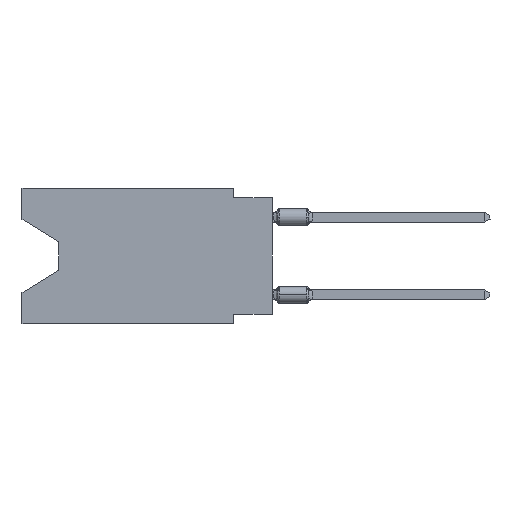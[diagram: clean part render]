
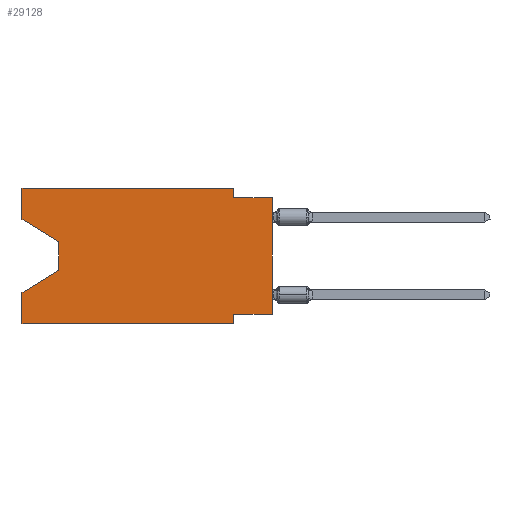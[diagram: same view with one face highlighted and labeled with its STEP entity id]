
A CAD part, left-side view. The second image highlights one B-rep face of the part: STEP entity #29128.
In plain terms, the highlighted planar face has unit normal (-1, 0, 0).
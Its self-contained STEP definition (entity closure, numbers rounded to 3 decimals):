
#544 = CARTESIAN_POINT ( 'NONE',  ( 0., 2.54, -8.89 ) ) ;
#2797 = DIRECTION ( 'NONE',  ( 0., 0., 1. ) ) ;
#3308 = CARTESIAN_POINT ( 'NONE',  ( 0., 0., -0.635 ) ) ;
#3754 = CARTESIAN_POINT ( 'NONE',  ( 0., 2.54, -8.255 ) ) ;
#3986 = CARTESIAN_POINT ( 'NONE',  ( 0., 2.54, -8.89 ) ) ;
#6310 = ORIENTED_EDGE ( 'NONE', *, *, #25514, .T. ) ;
#7129 = ORIENTED_EDGE ( 'NONE', *, *, #29962, .F. ) ;
#7246 = LINE ( 'NONE', #46745, #50646 ) ;
#7918 = VECTOR ( 'NONE', #38647, 1000. ) ;
#8728 = ORIENTED_EDGE ( 'NONE', *, *, #28057, .F. ) ;
#8748 = CARTESIAN_POINT ( 'NONE',  ( 0., 16.383, 0. ) ) ;
#9948 = DIRECTION ( 'NONE',  ( 0., -0.855, -0.519 ) ) ;
#12401 = ORIENTED_EDGE ( 'NONE', *, *, #23514, .T. ) ;
#13628 = CARTESIAN_POINT ( 'NONE',  ( 0., 13.97, -5.385 ) ) ;
#14386 = VECTOR ( 'NONE', #37994, 1000. ) ;
#14815 = VERTEX_POINT ( 'NONE', #20829 ) ;
#14848 = LINE ( 'NONE', #34780, #24782 ) ;
#15289 = EDGE_CURVE ( 'NONE', #25680, #18998, #44597, .T. ) ;
#16782 = VERTEX_POINT ( 'NONE', #3754 ) ;
#17355 = DIRECTION ( 'NONE',  ( 0., 0., 1. ) ) ;
#17491 = CARTESIAN_POINT ( 'NONE',  ( 0., 16.383, -8.89 ) ) ;
#18998 = VERTEX_POINT ( 'NONE', #3308 ) ;
#19132 = ORIENTED_EDGE ( 'NONE', *, *, #34079, .F. ) ;
#19628 = ORIENTED_EDGE ( 'NONE', *, *, #15289, .F. ) ;
#19960 = VECTOR ( 'NONE', #62646, 1000. ) ;
#20457 = DIRECTION ( 'NONE',  ( 0., 0., -1. ) ) ;
#20829 = CARTESIAN_POINT ( 'NONE',  ( 0., 16.383, -8.89 ) ) ;
#22309 = CARTESIAN_POINT ( 'NONE',  ( 0., 0., -8.255 ) ) ;
#22534 = CARTESIAN_POINT ( 'NONE',  ( 0., 0., -8.255 ) ) ;
#23514 = EDGE_CURVE ( 'NONE', #55334, #18998, #26099, .T. ) ;
#24268 = ORIENTED_EDGE ( 'NONE', *, *, #50638, .F. ) ;
#24782 = VECTOR ( 'NONE', #9948, 1000. ) ;
#24988 = CARTESIAN_POINT ( 'NONE',  ( 0., 16.383, -2.038 ) ) ;
#25101 = VECTOR ( 'NONE', #35912, 1000. ) ;
#25110 = LINE ( 'NONE', #17491, #61078 ) ;
#25514 = EDGE_CURVE ( 'NONE', #60971, #62952, #43201, .T. ) ;
#25680 = VERTEX_POINT ( 'NONE', #40229 ) ;
#26099 = LINE ( 'NONE', #62016, #25101 ) ;
#26554 = PLANE ( 'NONE',  #51861 ) ;
#27206 = DIRECTION ( 'NONE',  ( 0., 0., -1. ) ) ;
#27913 = ORIENTED_EDGE ( 'NONE', *, *, #57124, .F. ) ;
#27999 = LINE ( 'NONE', #8748, #52180 ) ;
#28057 = EDGE_CURVE ( 'NONE', #55334, #16782, #47112, .T. ) ;
#29037 = EDGE_CURVE ( 'NONE', #37709, #36708, #14848, .T. ) ;
#29128 = ADVANCED_FACE ( 'NONE', ( #46813 ), #26554, .F. ) ;
#29423 = CARTESIAN_POINT ( 'NONE',  ( 0., 16.383, 0. ) ) ;
#29962 = EDGE_CURVE ( 'NONE', #37709, #45222, #46222, .T. ) ;
#30205 = DIRECTION ( 'NONE',  ( 0., -1., 0. ) ) ;
#31523 = CARTESIAN_POINT ( 'NONE',  ( 0., 16.383, 0. ) ) ;
#32145 = EDGE_CURVE ( 'NONE', #45222, #53547, #27999, .T. ) ;
#32771 = CARTESIAN_POINT ( 'NONE',  ( 0., 16.383, -6.852 ) ) ;
#33240 = DIRECTION ( 'NONE',  ( 0., -1., 0. ) ) ;
#34079 = EDGE_CURVE ( 'NONE', #53547, #25680, #47617, .T. ) ;
#34780 = CARTESIAN_POINT ( 'NONE',  ( 0., 16.383, -2.038 ) ) ;
#35038 = VECTOR ( 'NONE', #17355, 1000. ) ;
#35664 = ORIENTED_EDGE ( 'NONE', *, *, #50561, .T. ) ;
#35912 = DIRECTION ( 'NONE',  ( 0., 0., 1. ) ) ;
#35940 = VECTOR ( 'NONE', #20457, 1000. ) ;
#36708 = VERTEX_POINT ( 'NONE', #44752 ) ;
#37709 = VERTEX_POINT ( 'NONE', #24988 ) ;
#37935 = LINE ( 'NONE', #52620, #35038 ) ;
#37994 = DIRECTION ( 'NONE',  ( 0., 1., 0. ) ) ;
#38647 = DIRECTION ( 'NONE',  ( 0., 0.855, -0.519 ) ) ;
#39609 = VERTEX_POINT ( 'NONE', #3986 ) ;
#40229 = CARTESIAN_POINT ( 'NONE',  ( 0., 2.54, -0.635 ) ) ;
#41081 = DIRECTION ( 'NONE',  ( 0., -1., 0. ) ) ;
#41629 = ORIENTED_EDGE ( 'NONE', *, *, #47003, .T. ) ;
#43131 = VECTOR ( 'NONE', #30205, 1000. ) ;
#43201 = LINE ( 'NONE', #63467, #7918 ) ;
#44597 = LINE ( 'NONE', #45230, #43131 ) ;
#44752 = CARTESIAN_POINT ( 'NONE',  ( 0., 13.97, -3.505 ) ) ;
#45222 = VERTEX_POINT ( 'NONE', #29423 ) ;
#45230 = CARTESIAN_POINT ( 'NONE',  ( 0., 0., -0.635 ) ) ;
#46222 = LINE ( 'NONE', #31523, #50927 ) ;
#46481 = CARTESIAN_POINT ( 'NONE',  ( 0., 16.383, 0. ) ) ;
#46745 = CARTESIAN_POINT ( 'NONE',  ( 0., 13.97, -3.505 ) ) ;
#46813 = FACE_OUTER_BOUND ( 'NONE', #56754, .T. ) ;
#47003 = EDGE_CURVE ( 'NONE', #14815, #39609, #25110, .T. ) ;
#47112 = LINE ( 'NONE', #22309, #14386 ) ;
#47382 = DIRECTION ( 'NONE',  ( 0., 0., -1. ) ) ;
#47617 = LINE ( 'NONE', #53834, #19960 ) ;
#50561 = EDGE_CURVE ( 'NONE', #36708, #60971, #7246, .T. ) ;
#50638 = EDGE_CURVE ( 'NONE', #14815, #62952, #37935, .T. ) ;
#50646 = VECTOR ( 'NONE', #47382, 1000. ) ;
#50927 = VECTOR ( 'NONE', #2797, 1000. ) ;
#51058 = ORIENTED_EDGE ( 'NONE', *, *, #32145, .F. ) ;
#51717 = DIRECTION ( 'NONE',  ( 1., 0., 0. ) ) ;
#51861 = AXIS2_PLACEMENT_3D ( 'NONE', #46481, #51717, #27206 ) ;
#52180 = VECTOR ( 'NONE', #33240, 1000. ) ;
#52620 = CARTESIAN_POINT ( 'NONE',  ( 0., 16.383, 0. ) ) ;
#53547 = VERTEX_POINT ( 'NONE', #59257 ) ;
#53834 = CARTESIAN_POINT ( 'NONE',  ( 0., 2.54, 0. ) ) ;
#54748 = LINE ( 'NONE', #544, #35940 ) ;
#55334 = VERTEX_POINT ( 'NONE', #22534 ) ;
#56754 = EDGE_LOOP ( 'NONE', ( #63371, #35664, #6310, #24268, #41629, #27913, #8728, #12401, #19628, #19132, #51058, #7129 ) ) ;
#57124 = EDGE_CURVE ( 'NONE', #16782, #39609, #54748, .T. ) ;
#59257 = CARTESIAN_POINT ( 'NONE',  ( 0., 2.54, 0. ) ) ;
#60971 = VERTEX_POINT ( 'NONE', #13628 ) ;
#61078 = VECTOR ( 'NONE', #41081, 1000. ) ;
#62016 = CARTESIAN_POINT ( 'NONE',  ( 0., 0., 0. ) ) ;
#62646 = DIRECTION ( 'NONE',  ( 0., 0., -1. ) ) ;
#62952 = VERTEX_POINT ( 'NONE', #32771 ) ;
#63371 = ORIENTED_EDGE ( 'NONE', *, *, #29037, .T. ) ;
#63467 = CARTESIAN_POINT ( 'NONE',  ( 0., 13.97, -5.385 ) ) ;
